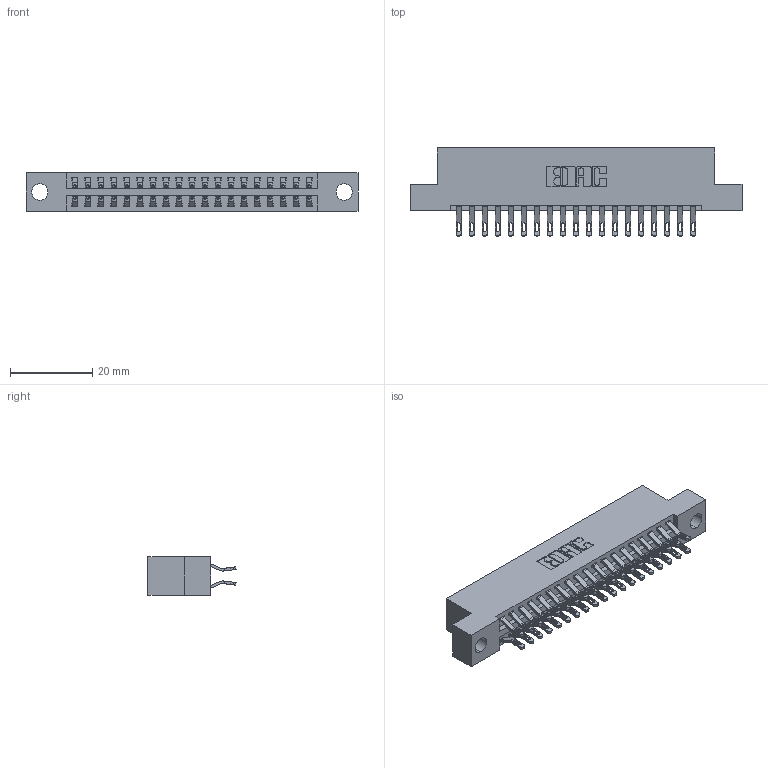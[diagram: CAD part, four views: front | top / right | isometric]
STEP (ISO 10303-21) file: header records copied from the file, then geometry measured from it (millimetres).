
FILE_DESCRIPTION (( 'STEP AP203' ), '1' );
FILE_NAME ('346-038-555-204.STEP', '2022-05-20T00:03:29', ( '' ), ( '' ), 'SwSTEP 2.0', 'SolidWorks 2020', '' );
FILE_SCHEMA (( 'CONFIG_CONTROL_DESIGN' ));
Length unit declared in the file: inch
Products named in the file (3): 346-038-555-204; 345-292-001_555 Tail; 346 Part_Flush Mounting Lugs - 0.156 Dia-TH
Assembly tree (39 placements, depth 2):
  346-038-555-204
    346 Part_Flush Mounting Lugs - 0.156 Dia-TH
    345-292-001_555 Tail  x38
Bounding box: 80.9 x 21.46 x 9.4 mm (x, y, z)
Volume: 7714.3 mm3; surface area: 10483.1 mm2
Topology: 39 solids, 39 shells, 2340 faces, 7319 edges, 4878 vertices
Faces by surface type: plane 1344, cylinder 996
Entity records: 16241 total; most frequent: CARTESIAN_POINT 2748, ORIENTED_EDGE 2650, DIRECTION 2441, EDGE_CURVE 1325, VECTOR 1097, LINE 1097, VERTEX_POINT 882, AXIS2_PLACEMENT_3D 672
